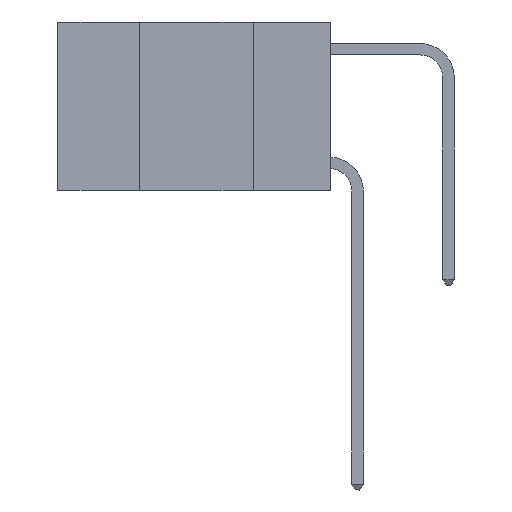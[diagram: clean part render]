
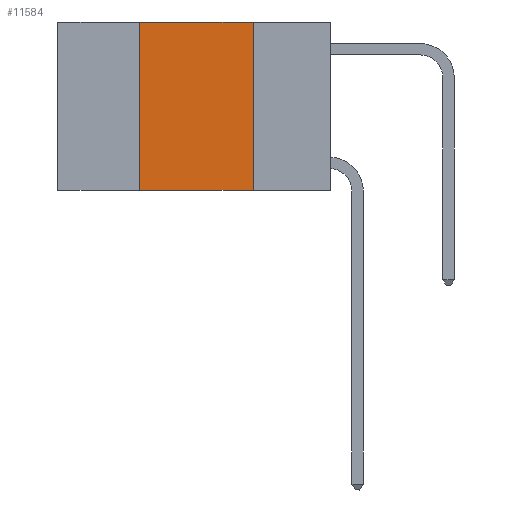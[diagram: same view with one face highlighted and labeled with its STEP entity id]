
A CAD part, left-side view. The second image highlights one B-rep face of the part: STEP entity #11584.
In plain terms, the highlighted planar face has unit normal (-1, 0, 0).
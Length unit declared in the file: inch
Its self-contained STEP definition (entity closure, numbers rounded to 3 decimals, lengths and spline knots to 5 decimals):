
#417 = EDGE_LOOP ( 'NONE', ( #22062, #10383, #13108, #23867 ) ) ;
#612 = VECTOR ( 'NONE', #7431, 39.37008 ) ;
#968 = EDGE_CURVE ( 'NONE', #1281, #4761, #7308, .T. ) ;
#1202 = CARTESIAN_POINT ( 'NONE',  ( 0., 0.17, -0.37 ) ) ;
#1246 = CARTESIAN_POINT ( 'NONE',  ( 0., 0.6, -0.37 ) ) ;
#1281 = VERTEX_POINT ( 'NONE', #13094 ) ;
#2216 = DIRECTION ( 'NONE',  ( 0., 0., 1. ) ) ;
#2372 = PLANE ( 'NONE',  #2875 ) ;
#2501 = CARTESIAN_POINT ( 'NONE',  ( 0., 0.6, 0. ) ) ;
#2855 = EDGE_CURVE ( 'NONE', #9260, #9994, #17011, .T. ) ;
#2875 = AXIS2_PLACEMENT_3D ( 'NONE', #2501, #12409, #18531 ) ;
#4761 = VERTEX_POINT ( 'NONE', #15310 ) ;
#6783 = FACE_OUTER_BOUND ( 'NONE', #417, .T. ) ;
#7308 = LINE ( 'NONE', #20896, #25636 ) ;
#7431 = DIRECTION ( 'NONE',  ( 0., -1., 0. ) ) ;
#9260 = VERTEX_POINT ( 'NONE', #18062 ) ;
#9994 = VERTEX_POINT ( 'NONE', #1202 ) ;
#10383 = ORIENTED_EDGE ( 'NONE', *, *, #968, .F. ) ;
#11584 = ADVANCED_FACE ( 'NONE', ( #6783 ), #2372, .F. ) ;
#12409 = DIRECTION ( 'NONE',  ( 1., 0., 0. ) ) ;
#12526 = CARTESIAN_POINT ( 'NONE',  ( 0., 0.17, 0. ) ) ;
#13094 = CARTESIAN_POINT ( 'NONE',  ( 0., 0.42, 0. ) ) ;
#13108 = ORIENTED_EDGE ( 'NONE', *, *, #25573, .F. ) ;
#15310 = CARTESIAN_POINT ( 'NONE',  ( 0., 0.17, 0. ) ) ;
#16115 = VECTOR ( 'NONE', #2216, 39.37008 ) ;
#16801 = VECTOR ( 'NONE', #20480, 39.37008 ) ;
#17011 = LINE ( 'NONE', #1246, #612 ) ;
#18062 = CARTESIAN_POINT ( 'NONE',  ( 0., 0.42, -0.37 ) ) ;
#18531 = DIRECTION ( 'NONE',  ( 0., 0., -1. ) ) ;
#18658 = EDGE_CURVE ( 'NONE', #4761, #9994, #18777, .T. ) ;
#18777 = LINE ( 'NONE', #12526, #16801 ) ;
#19792 = LINE ( 'NONE', #21904, #16115 ) ;
#20480 = DIRECTION ( 'NONE',  ( 0., 0., -1. ) ) ;
#20640 = DIRECTION ( 'NONE',  ( 0., -1., 0. ) ) ;
#20896 = CARTESIAN_POINT ( 'NONE',  ( 0., 0.6, 0. ) ) ;
#21904 = CARTESIAN_POINT ( 'NONE',  ( 0., 0.42, 0. ) ) ;
#22062 = ORIENTED_EDGE ( 'NONE', *, *, #18658, .F. ) ;
#23867 = ORIENTED_EDGE ( 'NONE', *, *, #2855, .T. ) ;
#25573 = EDGE_CURVE ( 'NONE', #9260, #1281, #19792, .T. ) ;
#25636 = VECTOR ( 'NONE', #20640, 39.37008 ) ;
